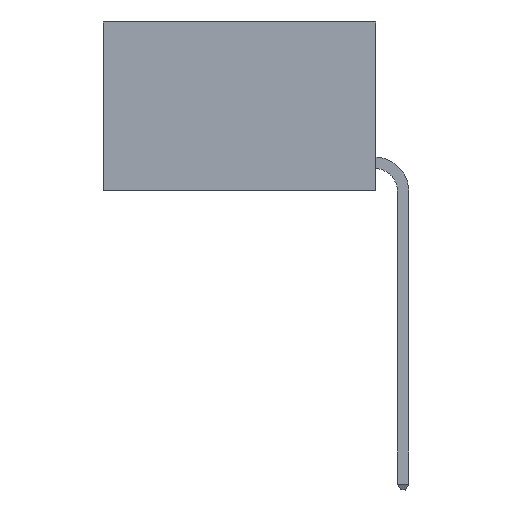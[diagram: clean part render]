
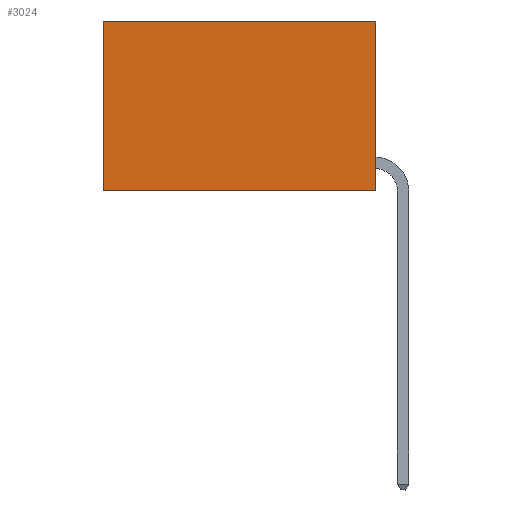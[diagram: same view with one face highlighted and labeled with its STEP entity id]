
A CAD part, left-side view. The second image highlights one B-rep face of the part: STEP entity #3024.
In plain terms, the highlighted planar face has unit normal (-1, 0, 0).
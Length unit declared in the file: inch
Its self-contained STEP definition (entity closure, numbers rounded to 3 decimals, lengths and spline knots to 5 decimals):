
#10 = PLANE ( 'NONE',  #439 ) ;
#132 = LINE ( 'NONE', #8682, #5223 ) ;
#198 = FACE_OUTER_BOUND ( 'NONE', #7669, .T. ) ;
#419 = VECTOR ( 'NONE', #8057, 39.37008 ) ;
#439 = AXIS2_PLACEMENT_3D ( 'NONE', #774, #1550, #6428 ) ;
#544 = CARTESIAN_POINT ( 'NONE',  ( 0.2625, 0., 0. ) ) ;
#765 = LINE ( 'NONE', #8196, #6195 ) ;
#774 = CARTESIAN_POINT ( 'NONE',  ( 0.2625, 0., 0. ) ) ;
#781 = EDGE_CURVE ( 'NONE', #4717, #5858, #2257, .T. ) ;
#914 = ORIENTED_EDGE ( 'NONE', *, *, #781, .T. ) ;
#1507 = VERTEX_POINT ( 'NONE', #4558 ) ;
#1550 = DIRECTION ( 'NONE',  ( 1., 0., 0. ) ) ;
#2021 = CARTESIAN_POINT ( 'NONE',  ( 0.2625, 0.6, 0. ) ) ;
#2078 = ORIENTED_EDGE ( 'NONE', *, *, #3361, .F. ) ;
#2257 = LINE ( 'NONE', #2021, #419 ) ;
#2703 = EDGE_CURVE ( 'NONE', #5426, #4717, #5083, .T. ) ;
#3024 = ADVANCED_FACE ( 'NONE', ( #198 ), #10, .F. ) ;
#3361 = EDGE_CURVE ( 'NONE', #5426, #1507, #765, .T. ) ;
#3650 = ORIENTED_EDGE ( 'NONE', *, *, #6340, .F. ) ;
#4558 = CARTESIAN_POINT ( 'NONE',  ( 0.2625, 0., -0.37 ) ) ;
#4672 = VECTOR ( 'NONE', #5446, 39.37008 ) ;
#4717 = VERTEX_POINT ( 'NONE', #6013 ) ;
#4860 = DIRECTION ( 'NONE',  ( 0., 1., 0. ) ) ;
#5083 = LINE ( 'NONE', #7361, #4672 ) ;
#5223 = VECTOR ( 'NONE', #4860, 39.37008 ) ;
#5426 = VERTEX_POINT ( 'NONE', #544 ) ;
#5446 = DIRECTION ( 'NONE',  ( 0., 1., 0. ) ) ;
#5858 = VERTEX_POINT ( 'NONE', #7120 ) ;
#5897 = ORIENTED_EDGE ( 'NONE', *, *, #2703, .T. ) ;
#6013 = CARTESIAN_POINT ( 'NONE',  ( 0.2625, 0.6, 0. ) ) ;
#6195 = VECTOR ( 'NONE', #8801, 39.37008 ) ;
#6340 = EDGE_CURVE ( 'NONE', #1507, #5858, #132, .T. ) ;
#6428 = DIRECTION ( 'NONE',  ( 0., 0., -1. ) ) ;
#7120 = CARTESIAN_POINT ( 'NONE',  ( 0.2625, 0.6, -0.37 ) ) ;
#7361 = CARTESIAN_POINT ( 'NONE',  ( 0.2625, 0., 0. ) ) ;
#7669 = EDGE_LOOP ( 'NONE', ( #914, #3650, #2078, #5897 ) ) ;
#8057 = DIRECTION ( 'NONE',  ( 0., 0., -1. ) ) ;
#8196 = CARTESIAN_POINT ( 'NONE',  ( 0.2625, 0., 0. ) ) ;
#8682 = CARTESIAN_POINT ( 'NONE',  ( 0.2625, 0., -0.37 ) ) ;
#8801 = DIRECTION ( 'NONE',  ( 0., 0., -1. ) ) ;
